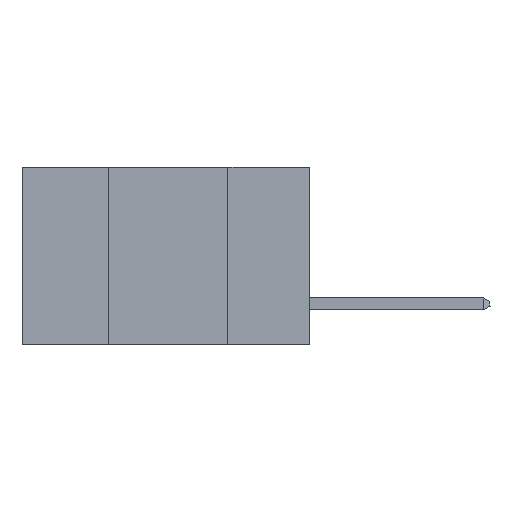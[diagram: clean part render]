
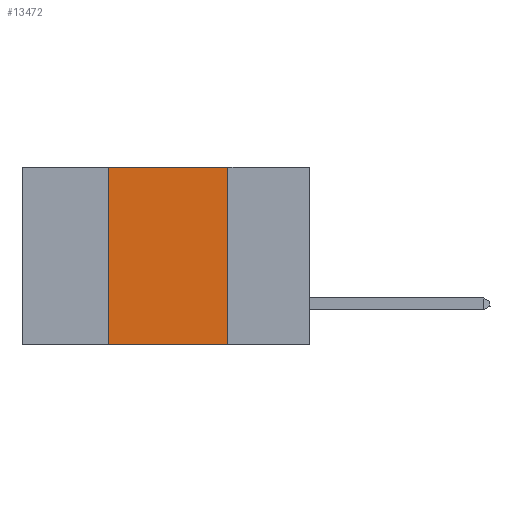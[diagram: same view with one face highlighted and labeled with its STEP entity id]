
A CAD part, left-side view. The second image highlights one B-rep face of the part: STEP entity #13472.
In plain terms, the highlighted planar face has unit normal (-1, 0, 0).
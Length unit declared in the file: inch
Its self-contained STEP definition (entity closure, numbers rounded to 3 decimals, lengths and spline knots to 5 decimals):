
#1973 = EDGE_CURVE ( 'NONE', #19385, #22999, #5588, .T. ) ;
#2777 = EDGE_CURVE ( 'NONE', #8547, #19385, #17106, .T. ) ;
#4571 = CARTESIAN_POINT ( 'NONE',  ( 0., 0.6, -0.37 ) ) ;
#4678 = ORIENTED_EDGE ( 'NONE', *, *, #15937, .F. ) ;
#5086 = CARTESIAN_POINT ( 'NONE',  ( 0., 0.42, -0.37 ) ) ;
#5588 = LINE ( 'NONE', #26252, #27946 ) ;
#5710 = PLANE ( 'NONE',  #8107 ) ;
#5811 = CARTESIAN_POINT ( 'NONE',  ( 0., 0.6, 0. ) ) ;
#7304 = CARTESIAN_POINT ( 'NONE',  ( 0., 0.17, 0. ) ) ;
#7783 = LINE ( 'NONE', #10717, #11824 ) ;
#7839 = ORIENTED_EDGE ( 'NONE', *, *, #1973, .F. ) ;
#7996 = DIRECTION ( 'NONE',  ( 1., 0., 0. ) ) ;
#8107 = AXIS2_PLACEMENT_3D ( 'NONE', #5811, #7996, #25063 ) ;
#8547 = VERTEX_POINT ( 'NONE', #5086 ) ;
#8754 = DIRECTION ( 'NONE',  ( 0., -1., 0. ) ) ;
#10717 = CARTESIAN_POINT ( 'NONE',  ( 0., 0.17, 0. ) ) ;
#11509 = DIRECTION ( 'NONE',  ( 0., 0., 1. ) ) ;
#11538 = LINE ( 'NONE', #4571, #21419 ) ;
#11824 = VECTOR ( 'NONE', #19905, 39.37008 ) ;
#13472 = ADVANCED_FACE ( 'NONE', ( #14044 ), #5710, .F. ) ;
#13624 = CARTESIAN_POINT ( 'NONE',  ( 0., 0.42, 0. ) ) ;
#14044 = FACE_OUTER_BOUND ( 'NONE', #23321, .T. ) ;
#15348 = EDGE_CURVE ( 'NONE', #8547, #20616, #11538, .T. ) ;
#15937 = EDGE_CURVE ( 'NONE', #22999, #20616, #7783, .T. ) ;
#17106 = LINE ( 'NONE', #25915, #24222 ) ;
#17646 = DIRECTION ( 'NONE',  ( 0., -1., 0. ) ) ;
#19385 = VERTEX_POINT ( 'NONE', #13624 ) ;
#19905 = DIRECTION ( 'NONE',  ( 0., 0., -1. ) ) ;
#20011 = ORIENTED_EDGE ( 'NONE', *, *, #15348, .T. ) ;
#20616 = VERTEX_POINT ( 'NONE', #24751 ) ;
#21419 = VECTOR ( 'NONE', #8754, 39.37008 ) ;
#22999 = VERTEX_POINT ( 'NONE', #7304 ) ;
#23321 = EDGE_LOOP ( 'NONE', ( #4678, #7839, #23568, #20011 ) ) ;
#23568 = ORIENTED_EDGE ( 'NONE', *, *, #2777, .F. ) ;
#24222 = VECTOR ( 'NONE', #11509, 39.37008 ) ;
#24751 = CARTESIAN_POINT ( 'NONE',  ( 0., 0.17, -0.37 ) ) ;
#25063 = DIRECTION ( 'NONE',  ( 0., 0., -1. ) ) ;
#25915 = CARTESIAN_POINT ( 'NONE',  ( 0., 0.42, 0. ) ) ;
#26252 = CARTESIAN_POINT ( 'NONE',  ( 0., 0.6, 0. ) ) ;
#27946 = VECTOR ( 'NONE', #17646, 39.37008 ) ;
